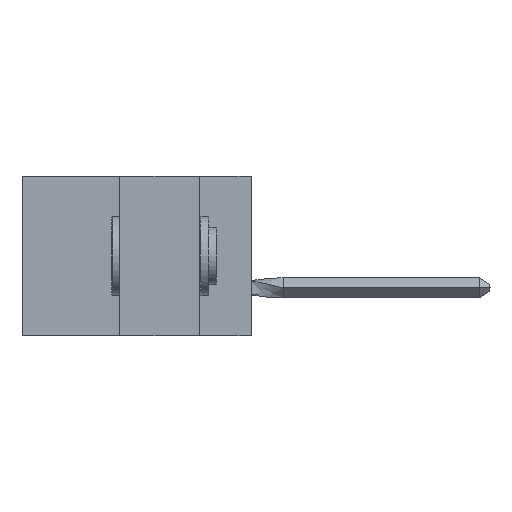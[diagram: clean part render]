
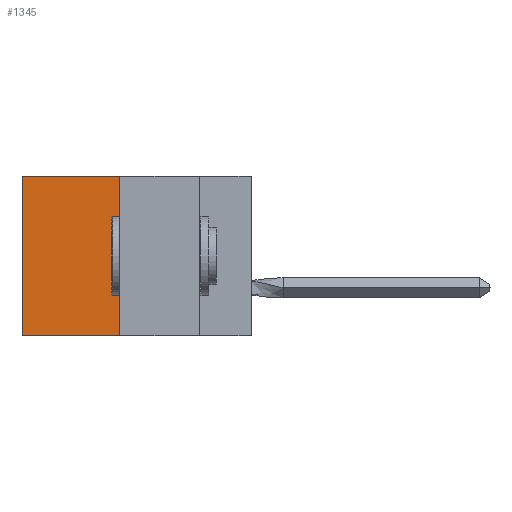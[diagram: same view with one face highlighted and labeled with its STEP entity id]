
A CAD part, left-side view. The second image highlights one B-rep face of the part: STEP entity #1345.
In plain terms, the highlighted planar face has unit normal (-1, 0, 0).
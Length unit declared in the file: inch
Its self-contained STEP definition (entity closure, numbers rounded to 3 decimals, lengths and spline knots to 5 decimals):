
#1345 = ADVANCED_FACE ( 'NONE', ( #26809 ), #31985, .F. ) ;
#1373 = VECTOR ( 'NONE', #19061, 39.37008 ) ;
#1456 = CARTESIAN_POINT ( 'NONE',  ( 0.305, 0.413, -0.5 ) ) ;
#2476 = VECTOR ( 'NONE', #5757, 39.37008 ) ;
#3232 = LINE ( 'NONE', #12983, #10503 ) ;
#5757 = DIRECTION ( 'NONE',  ( 0., 1., 0. ) ) ;
#6673 = DIRECTION ( 'NONE',  ( 0., 1., 0. ) ) ;
#8815 = DIRECTION ( 'NONE',  ( 0., 0., -1. ) ) ;
#10503 = VECTOR ( 'NONE', #24179, 39.37008 ) ;
#11039 = LINE ( 'NONE', #18453, #21444 ) ;
#12983 = CARTESIAN_POINT ( 'NONE',  ( 0.305, 0.72, -0.5 ) ) ;
#14108 = CARTESIAN_POINT ( 'NONE',  ( 0.305, 0.413, 0. ) ) ;
#15107 = ORIENTED_EDGE ( 'NONE', *, *, #16600, .F. ) ;
#15453 = VERTEX_POINT ( 'NONE', #28021 ) ;
#16600 = EDGE_CURVE ( 'NONE', #28549, #32461, #11039, .T. ) ;
#17646 = DIRECTION ( 'NONE',  ( 1., 0., 0. ) ) ;
#18453 = CARTESIAN_POINT ( 'NONE',  ( 0.305, 0.413, -0.5 ) ) ;
#18583 = AXIS2_PLACEMENT_3D ( 'NONE', #20531, #17646, #8815 ) ;
#18767 = EDGE_LOOP ( 'NONE', ( #21066, #15107, #27137, #23505 ) ) ;
#18905 = EDGE_CURVE ( 'NONE', #31175, #28549, #23098, .T. ) ;
#19061 = DIRECTION ( 'NONE',  ( 0., 0., -1. ) ) ;
#20531 = CARTESIAN_POINT ( 'NONE',  ( 0.305, 0.413, -0.5 ) ) ;
#21066 = ORIENTED_EDGE ( 'NONE', *, *, #32840, .T. ) ;
#21444 = VECTOR ( 'NONE', #6673, 39.37008 ) ;
#22453 = CARTESIAN_POINT ( 'NONE',  ( 0.305, 0.72, -0.5 ) ) ;
#23098 = LINE ( 'NONE', #1456, #1373 ) ;
#23505 = ORIENTED_EDGE ( 'NONE', *, *, #34370, .T. ) ;
#24179 = DIRECTION ( 'NONE',  ( 0., 0., -1. ) ) ;
#26809 = FACE_OUTER_BOUND ( 'NONE', #18767, .T. ) ;
#27077 = CARTESIAN_POINT ( 'NONE',  ( 0.305, 0.413, -0.5 ) ) ;
#27137 = ORIENTED_EDGE ( 'NONE', *, *, #18905, .F. ) ;
#27832 = CARTESIAN_POINT ( 'NONE',  ( 0.305, 0.413, 0. ) ) ;
#28021 = CARTESIAN_POINT ( 'NONE',  ( 0.305, 0.72, 0. ) ) ;
#28549 = VERTEX_POINT ( 'NONE', #27077 ) ;
#31175 = VERTEX_POINT ( 'NONE', #27832 ) ;
#31985 = PLANE ( 'NONE',  #18583 ) ;
#32461 = VERTEX_POINT ( 'NONE', #22453 ) ;
#32840 = EDGE_CURVE ( 'NONE', #15453, #32461, #3232, .T. ) ;
#34370 = EDGE_CURVE ( 'NONE', #31175, #15453, #37217, .T. ) ;
#37217 = LINE ( 'NONE', #14108, #2476 ) ;
